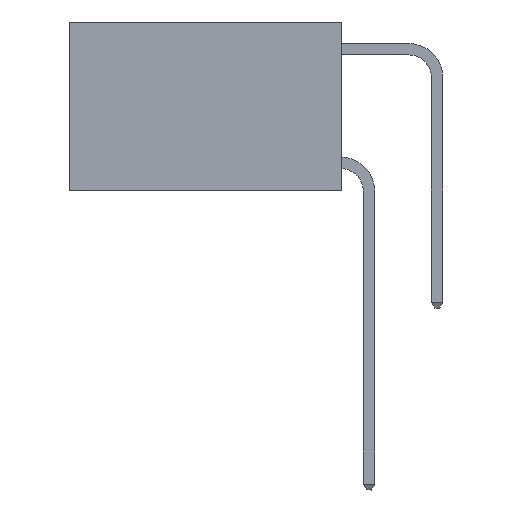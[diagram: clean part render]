
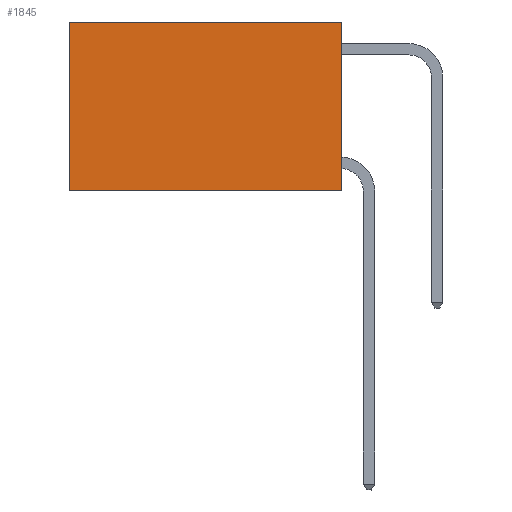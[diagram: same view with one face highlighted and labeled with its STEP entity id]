
A CAD part, left-side view. The second image highlights one B-rep face of the part: STEP entity #1845.
In plain terms, the highlighted planar face has unit normal (-1, 0, 0).
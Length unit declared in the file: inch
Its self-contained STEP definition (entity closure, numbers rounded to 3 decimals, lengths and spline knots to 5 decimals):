
#552 = DIRECTION ( 'NONE',  ( 0., 0., -1. ) ) ;
#680 = FACE_OUTER_BOUND ( 'NONE', #1421, .T. ) ;
#731 = CARTESIAN_POINT ( 'NONE',  ( 0.2625, 0., 0. ) ) ;
#1171 = CARTESIAN_POINT ( 'NONE',  ( 0.2625, 0.6, -0.37 ) ) ;
#1421 = EDGE_LOOP ( 'NONE', ( #7738, #8877, #8542, #3152 ) ) ;
#1459 = VECTOR ( 'NONE', #11984, 39.37008 ) ;
#1845 = ADVANCED_FACE ( 'NONE', ( #680 ), #7642, .F. ) ;
#2207 = CARTESIAN_POINT ( 'NONE',  ( 0.2625, 0., -0.37 ) ) ;
#2231 = CARTESIAN_POINT ( 'NONE',  ( 0.2625, 0., 0. ) ) ;
#2741 = CARTESIAN_POINT ( 'NONE',  ( 0.2625, 0.6, 0. ) ) ;
#3152 = ORIENTED_EDGE ( 'NONE', *, *, #14780, .T. ) ;
#3199 = VERTEX_POINT ( 'NONE', #2741 ) ;
#4143 = DIRECTION ( 'NONE',  ( 0., 0., -1. ) ) ;
#4679 = EDGE_CURVE ( 'NONE', #3199, #7034, #14016, .T. ) ;
#4853 = AXIS2_PLACEMENT_3D ( 'NONE', #731, #10881, #11830 ) ;
#4995 = LINE ( 'NONE', #9753, #1459 ) ;
#5372 = CARTESIAN_POINT ( 'NONE',  ( 0.2625, 0.6, 0. ) ) ;
#5661 = VECTOR ( 'NONE', #552, 39.37008 ) ;
#7034 = VERTEX_POINT ( 'NONE', #1171 ) ;
#7137 = VECTOR ( 'NONE', #4143, 39.37008 ) ;
#7642 = PLANE ( 'NONE',  #4853 ) ;
#7738 = ORIENTED_EDGE ( 'NONE', *, *, #4679, .T. ) ;
#8542 = ORIENTED_EDGE ( 'NONE', *, *, #9168, .F. ) ;
#8877 = ORIENTED_EDGE ( 'NONE', *, *, #14408, .F. ) ;
#9168 = EDGE_CURVE ( 'NONE', #9418, #9678, #9516, .T. ) ;
#9188 = LINE ( 'NONE', #2231, #12527 ) ;
#9418 = VERTEX_POINT ( 'NONE', #14370 ) ;
#9516 = LINE ( 'NONE', #11075, #7137 ) ;
#9678 = VERTEX_POINT ( 'NONE', #2207 ) ;
#9753 = CARTESIAN_POINT ( 'NONE',  ( 0.2625, 0., -0.37 ) ) ;
#10881 = DIRECTION ( 'NONE',  ( 1., 0., 0. ) ) ;
#11075 = CARTESIAN_POINT ( 'NONE',  ( 0.2625, 0., 0. ) ) ;
#11830 = DIRECTION ( 'NONE',  ( 0., 0., -1. ) ) ;
#11984 = DIRECTION ( 'NONE',  ( 0., 1., 0. ) ) ;
#12527 = VECTOR ( 'NONE', #13752, 39.37008 ) ;
#13752 = DIRECTION ( 'NONE',  ( 0., 1., 0. ) ) ;
#14016 = LINE ( 'NONE', #5372, #5661 ) ;
#14370 = CARTESIAN_POINT ( 'NONE',  ( 0.2625, 0., 0. ) ) ;
#14408 = EDGE_CURVE ( 'NONE', #9678, #7034, #4995, .T. ) ;
#14780 = EDGE_CURVE ( 'NONE', #9418, #3199, #9188, .T. ) ;
